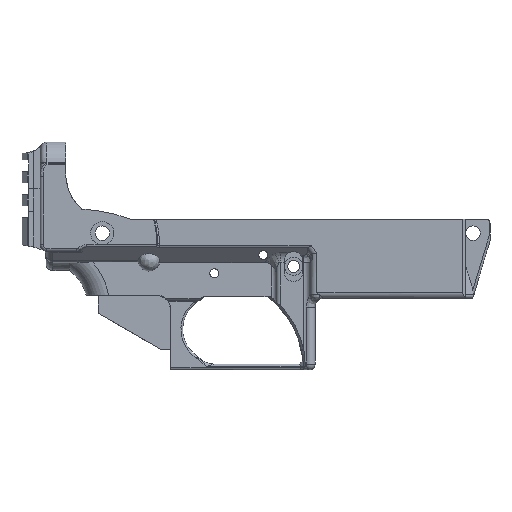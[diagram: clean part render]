
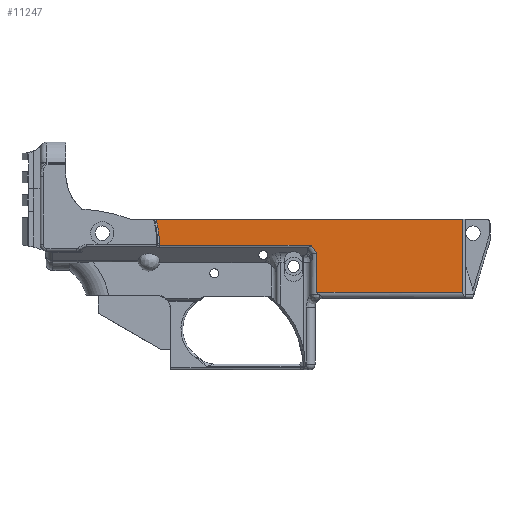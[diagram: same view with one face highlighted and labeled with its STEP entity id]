
A CAD part, left-side view. The second image highlights one B-rep face of the part: STEP entity #11247.
In plain terms, the highlighted planar face has unit normal (-1, 0, 0).
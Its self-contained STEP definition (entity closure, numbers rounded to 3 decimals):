
#115=ELLIPSE('',#12096,48.772,41.553);
#116=ELLIPSE('',#12097,3.231,2.315);
#1536=FACE_OUTER_BOUND('',#2177,.T.);
#2177=EDGE_LOOP('',(#10382,#10383,#10384,#10385,#10386,#10387,#10388,#10389));
#2896=LINE('',#24219,#3719);
#2926=LINE('',#25048,#3749);
#2930=LINE('',#25063,#3753);
#2942=LINE('',#25346,#3765);
#2945=LINE('',#25426,#3768);
#2995=LINE('',#28122,#3818);
#3719=VECTOR('',#14563,154.067);
#3749=VECTOR('',#14671,10.);
#3753=VECTOR('',#14681,10.);
#3765=VECTOR('',#14717,10.);
#3768=VECTOR('',#14722,53.92);
#3818=VECTOR('',#14986,34.547);
#5109=VERTEX_POINT('',#24216);
#5110=VERTEX_POINT('',#24218);
#5158=VERTEX_POINT('',#24701);
#5159=VERTEX_POINT('',#24814);
#5174=VERTEX_POINT('',#25039);
#5176=VERTEX_POINT('',#25047);
#5192=VERTEX_POINT('',#25107);
#5195=VERTEX_POINT('',#25344);
#6686=EDGE_CURVE('',#5109,#5110,#2896,.T.);
#6750=EDGE_CURVE('',#5158,#5109,#115,.T.);
#6752=EDGE_CURVE('',#5159,#5158,#116,.T.);
#6772=EDGE_CURVE('',#5174,#5176,#2926,.T.);
#6778=EDGE_CURVE('',#5176,#5159,#2930,.T.);
#6801=EDGE_CURVE('',#5195,#5192,#2942,.T.);
#6807=EDGE_CURVE('',#5192,#5174,#2945,.T.);
#6974=EDGE_CURVE('',#5110,#5195,#2995,.T.);
#10382=ORIENTED_EDGE('',*,*,#6807,.F.);
#10383=ORIENTED_EDGE('',*,*,#6801,.F.);
#10384=ORIENTED_EDGE('',*,*,#6974,.F.);
#10385=ORIENTED_EDGE('',*,*,#6686,.F.);
#10386=ORIENTED_EDGE('',*,*,#6750,.F.);
#10387=ORIENTED_EDGE('',*,*,#6752,.F.);
#10388=ORIENTED_EDGE('',*,*,#6778,.F.);
#10389=ORIENTED_EDGE('',*,*,#6772,.F.);
#10635=PLANE('',#12239);
#11247=ADVANCED_FACE('',(#1536),#10635,.F.);
#12096=AXIS2_PLACEMENT_3D('',#24703,#14647,#14648);
#12097=AXIS2_PLACEMENT_3D('',#24864,#14649,#14650);
#12239=AXIS2_PLACEMENT_3D('',#28544,#15019,#15020);
#14563=DIRECTION('',(0.,-1.,0.));
#14647=DIRECTION('center_axis',(-1.,0.,0.));
#14648=DIRECTION('ref_axis',(0.,0.179,-0.984));
#14649=DIRECTION('center_axis',(-1.,0.,0.));
#14650=DIRECTION('ref_axis',(0.,0.938,-0.347));
#14671=DIRECTION('',(0.,0.577,0.816));
#14681=DIRECTION('',(0.,1.,0.));
#14717=DIRECTION('',(0.,1.,0.));
#14722=DIRECTION('',(0.,0.,1.));
#14986=DIRECTION('',(0.,0.,-1.));
#15019=DIRECTION('center_axis',(1.,0.,0.));
#15020=DIRECTION('ref_axis',(0.,0.,-1.));
#24216=CARTESIAN_POINT('',(-18.567,14.676,-47.419));
#24218=CARTESIAN_POINT('',(-18.567,-119.209,-47.419));
#24219=CARTESIAN_POINT('',(-18.567,34.858,-47.419));
#24701=CARTESIAN_POINT('',(-18.567,13.248,-57.945));
#24703=CARTESIAN_POINT('Origin',(-18.567,55.012,-62.807));
#24814=CARTESIAN_POINT('',(-18.567,13.395,-58.763));
#24864=CARTESIAN_POINT('Origin',(-18.567,16.382,-58.541));
#25039=CARTESIAN_POINT('',(-18.567,-55.482,-62.313));
#25047=CARTESIAN_POINT('',(-18.567,-52.972,-58.763));
#25048=CARTESIAN_POINT('',(-18.567,-37.405,-36.748));
#25063=CARTESIAN_POINT('',(-18.567,59.659,-58.763));
#25107=CARTESIAN_POINT('',(-18.567,-55.482,-79.427));
#25344=CARTESIAN_POINT('',(-18.567,-119.209,-79.427));
#25346=CARTESIAN_POINT('',(-18.567,-37.862,-79.427));
#25426=CARTESIAN_POINT('',(-18.567,-55.482,-59.289));
#28122=CARTESIAN_POINT('',(-18.567,-119.209,-47.419));
#28544=CARTESIAN_POINT('Origin',(-18.567,-52.267,-63.423));
